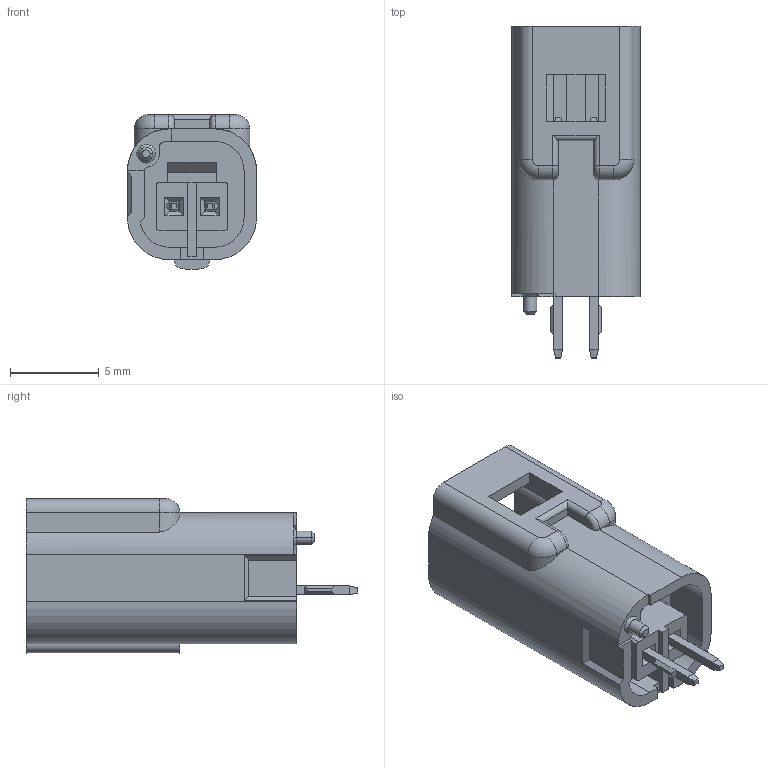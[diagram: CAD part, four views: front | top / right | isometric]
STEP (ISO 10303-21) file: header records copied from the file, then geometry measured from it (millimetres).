
FILE_DESCRIPTION (( 'STEP AP214' ), '1' );
FILE_NAME ('566-002-421-701.STEP', '2020-07-30T20:25:52', ( '' ), ( '' ), 'SwSTEP 2.0', 'SolidWorks 2020', '' );
FILE_SCHEMA (( 'AUTOMOTIVE_DESIGN' ));
Length unit declared in the file: millimetre
Products named in the file (5): 566-002-421-701; 566-002-421-701.STEP; 566-002-421-701_ rubber.STEP; contact.STEP; 566-002-421-701_plastic.STEP
Assembly tree (5 placements, depth 3):
  566-002-421-701
    566-002-421-701.STEP
      566-002-421-701_plastic.STEP
      566-002-421-701_ rubber.STEP
      contact.STEP  x2
Bounding box: 7.25 x 18.65 x 8.7 mm (x, y, z)
Volume: 393.9 mm3; surface area: 1195.1 mm2
Topology: 5 solids, 5 shells, 594 faces, 1420 edges, 856 vertices
Faces by surface type: plane 305, cylinder 193, torus 78, cone 18
Entity records: 15610 total; most frequent: DIRECTION 2791, CARTESIAN_POINT 2779, ORIENTED_EDGE 2564, EDGE_CURVE 1282, AXIS2_PLACEMENT_3D 994, VECTOR 803, LINE 803, VERTEX_POINT 768
